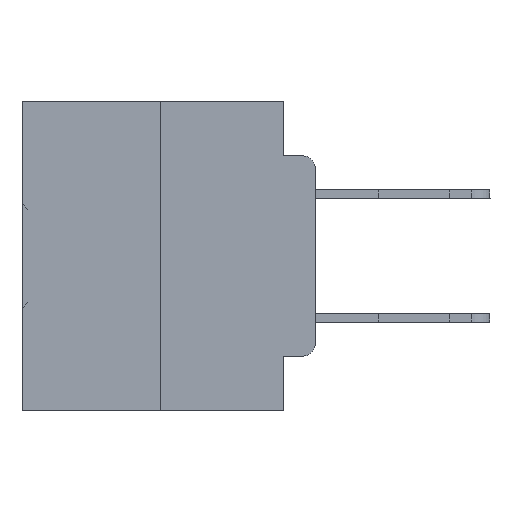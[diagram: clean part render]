
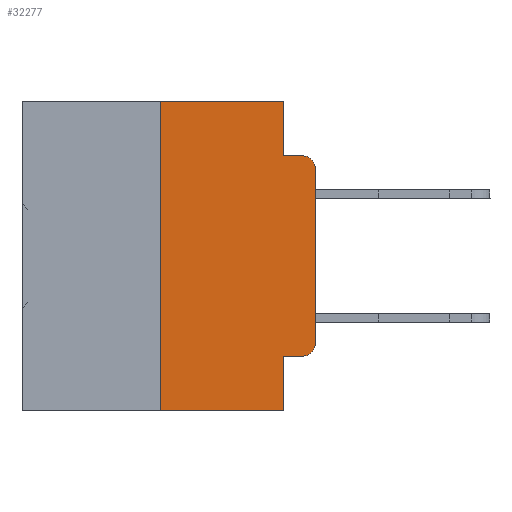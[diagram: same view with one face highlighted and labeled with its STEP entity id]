
A CAD part, left-side view. The second image highlights one B-rep face of the part: STEP entity #32277.
In plain terms, the highlighted planar face has unit normal (-1, 0, 0).
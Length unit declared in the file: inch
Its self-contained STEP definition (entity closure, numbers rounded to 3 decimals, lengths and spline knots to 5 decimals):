
#242 = VECTOR ( 'NONE', #1409, 39.37008 ) ;
#652 = CARTESIAN_POINT ( 'NONE',  ( 0., 0.02, -0.1085 ) ) ;
#747 = VECTOR ( 'NONE', #24716, 39.37008 ) ;
#797 = DIRECTION ( 'NONE',  ( 0., 0., -1. ) ) ;
#836 = DIRECTION ( 'NONE',  ( 0., 0., -1. ) ) ;
#868 = DIRECTION ( 'NONE',  ( 0., -1., 0. ) ) ;
#1102 = CARTESIAN_POINT ( 'NONE',  ( 0., 0.051, 0. ) ) ;
#1409 = DIRECTION ( 'NONE',  ( 0., -1., 0. ) ) ;
#1879 = ORIENTED_EDGE ( 'NONE', *, *, #5378, .T. ) ;
#2085 = VECTOR ( 'NONE', #19058, 39.37008 ) ;
#2301 = EDGE_CURVE ( 'NONE', #12486, #28209, #12954, .T. ) ;
#2946 = ORIENTED_EDGE ( 'NONE', *, *, #18459, .F. ) ;
#3223 = VERTEX_POINT ( 'NONE', #26729 ) ;
#3351 = CARTESIAN_POINT ( 'NONE',  ( 0., 0.051, -0.5 ) ) ;
#3412 = ORIENTED_EDGE ( 'NONE', *, *, #2301, .T. ) ;
#3756 = CARTESIAN_POINT ( 'NONE',  ( 0., 0.02, -0.4115 ) ) ;
#4096 = ORIENTED_EDGE ( 'NONE', *, *, #32385, .F. ) ;
#4576 = CARTESIAN_POINT ( 'NONE',  ( 0., 0., -0.1085 ) ) ;
#4756 = ORIENTED_EDGE ( 'NONE', *, *, #16853, .T. ) ;
#5097 = CARTESIAN_POINT ( 'NONE',  ( 0., 0.051, 0. ) ) ;
#5378 = EDGE_CURVE ( 'NONE', #34141, #12486, #35625, .T. ) ;
#5499 = VERTEX_POINT ( 'NONE', #15942 ) ;
#5701 = EDGE_CURVE ( 'NONE', #7200, #34141, #35814, .T. ) ;
#6013 = LINE ( 'NONE', #20260, #21226 ) ;
#6669 = DIRECTION ( 'NONE',  ( 0., -1., 0. ) ) ;
#7200 = VERTEX_POINT ( 'NONE', #9417 ) ;
#7324 = DIRECTION ( 'NONE',  ( 1., 0., 0. ) ) ;
#7513 = DIRECTION ( 'NONE',  ( 0., 0., -1. ) ) ;
#7623 = VERTEX_POINT ( 'NONE', #9552 ) ;
#7766 = CARTESIAN_POINT ( 'NONE',  ( 0., 0.02, -0.3915 ) ) ;
#9245 = ORIENTED_EDGE ( 'NONE', *, *, #14223, .F. ) ;
#9417 = CARTESIAN_POINT ( 'NONE',  ( 0., 0.051, -0.4115 ) ) ;
#9552 = CARTESIAN_POINT ( 'NONE',  ( 0., 0.25, 0. ) ) ;
#9560 = DIRECTION ( 'NONE',  ( 0., 0., -1. ) ) ;
#10185 = EDGE_CURVE ( 'NONE', #5499, #7623, #15258, .T. ) ;
#10217 = VECTOR ( 'NONE', #6669, 39.37008 ) ;
#10565 = DIRECTION ( 'NONE',  ( -1., 0., 0. ) ) ;
#11968 = ORIENTED_EDGE ( 'NONE', *, *, #26241, .T. ) ;
#12410 = CARTESIAN_POINT ( 'NONE',  ( 0., 0.473, -0.5 ) ) ;
#12486 = VERTEX_POINT ( 'NONE', #15935 ) ;
#12560 = ORIENTED_EDGE ( 'NONE', *, *, #10185, .F. ) ;
#12954 = LINE ( 'NONE', #15927, #2085 ) ;
#14223 = EDGE_CURVE ( 'NONE', #22084, #3223, #35309, .T. ) ;
#14363 = DIRECTION ( 'NONE',  ( 0., 0., -1. ) ) ;
#15258 = LINE ( 'NONE', #29485, #32851 ) ;
#15300 = CARTESIAN_POINT ( 'NONE',  ( 0., 0.473, 0. ) ) ;
#15741 = VECTOR ( 'NONE', #7513, 39.37008 ) ;
#15927 = CARTESIAN_POINT ( 'NONE',  ( 0., 0., 0. ) ) ;
#15935 = CARTESIAN_POINT ( 'NONE',  ( 0., 0., -0.3915 ) ) ;
#15942 = CARTESIAN_POINT ( 'NONE',  ( 0., 0.25, -0.5 ) ) ;
#16036 = CARTESIAN_POINT ( 'NONE',  ( 0., 0.051, -0.4115 ) ) ;
#16853 = EDGE_CURVE ( 'NONE', #5499, #22762, #23347, .T. ) ;
#17790 = AXIS2_PLACEMENT_3D ( 'NONE', #652, #20485, #9560 ) ;
#18459 = EDGE_CURVE ( 'NONE', #7623, #30771, #35092, .T. ) ;
#19058 = DIRECTION ( 'NONE',  ( 0., 0., 1. ) ) ;
#20260 = CARTESIAN_POINT ( 'NONE',  ( 0., 0.051, 0. ) ) ;
#20485 = DIRECTION ( 'NONE',  ( -1., 0., 0. ) ) ;
#20850 = AXIS2_PLACEMENT_3D ( 'NONE', #7766, #10565, #14363 ) ;
#21026 = LINE ( 'NONE', #5097, #15741 ) ;
#21226 = VECTOR ( 'NONE', #797, 39.37008 ) ;
#22084 = VERTEX_POINT ( 'NONE', #22649 ) ;
#22649 = CARTESIAN_POINT ( 'NONE',  ( 0., 0.051, -0.0885 ) ) ;
#22762 = VERTEX_POINT ( 'NONE', #3351 ) ;
#23347 = LINE ( 'NONE', #12410, #10217 ) ;
#24716 = DIRECTION ( 'NONE',  ( 0., -1., 0. ) ) ;
#25196 = AXIS2_PLACEMENT_3D ( 'NONE', #15300, #7324, #836 ) ;
#25772 = ORIENTED_EDGE ( 'NONE', *, *, #5701, .T. ) ;
#26203 = FACE_OUTER_BOUND ( 'NONE', #36151, .T. ) ;
#26235 = CARTESIAN_POINT ( 'NONE',  ( 0., 0.051, -0.0885 ) ) ;
#26241 = EDGE_CURVE ( 'NONE', #28209, #3223, #31889, .T. ) ;
#26538 = DIRECTION ( 'NONE',  ( 0., 0., 1. ) ) ;
#26729 = CARTESIAN_POINT ( 'NONE',  ( 0., 0.02, -0.0885 ) ) ;
#28209 = VERTEX_POINT ( 'NONE', #4576 ) ;
#29485 = CARTESIAN_POINT ( 'NONE',  ( 0., 0.25, 0. ) ) ;
#29710 = PLANE ( 'NONE',  #25196 ) ;
#30630 = ORIENTED_EDGE ( 'NONE', *, *, #35275, .F. ) ;
#30771 = VERTEX_POINT ( 'NONE', #1102 ) ;
#31889 = CIRCLE ( 'NONE', #17790, 0.02 ) ;
#32149 = CARTESIAN_POINT ( 'NONE',  ( 0., 0.473, 0. ) ) ;
#32277 = ADVANCED_FACE ( 'NONE', ( #26203 ), #29710, .F. ) ;
#32385 = EDGE_CURVE ( 'NONE', #7200, #22762, #21026, .T. ) ;
#32851 = VECTOR ( 'NONE', #26538, 39.37008 ) ;
#34141 = VERTEX_POINT ( 'NONE', #3756 ) ;
#34171 = VECTOR ( 'NONE', #868, 39.37008 ) ;
#35092 = LINE ( 'NONE', #32149, #242 ) ;
#35275 = EDGE_CURVE ( 'NONE', #30771, #22084, #6013, .T. ) ;
#35309 = LINE ( 'NONE', #26235, #34171 ) ;
#35625 = CIRCLE ( 'NONE', #20850, 0.02 ) ;
#35814 = LINE ( 'NONE', #16036, #747 ) ;
#36151 = EDGE_LOOP ( 'NONE', ( #3412, #11968, #9245, #30630, #2946, #12560, #4756, #4096, #25772, #1879 ) ) ;
